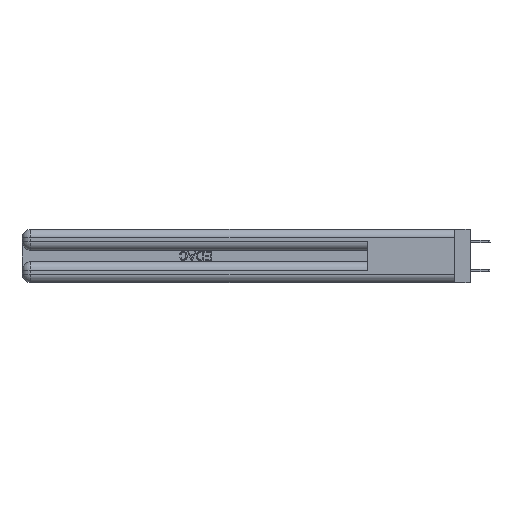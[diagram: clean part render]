
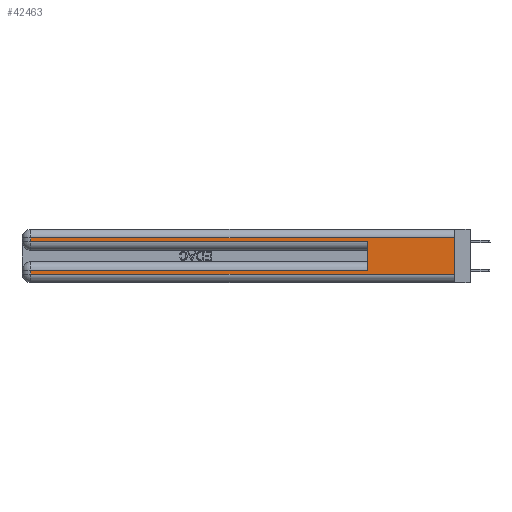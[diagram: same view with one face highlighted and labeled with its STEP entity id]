
A CAD part, left-side view. The second image highlights one B-rep face of the part: STEP entity #42463.
In plain terms, the highlighted planar face has unit normal (-1, 0, 0).
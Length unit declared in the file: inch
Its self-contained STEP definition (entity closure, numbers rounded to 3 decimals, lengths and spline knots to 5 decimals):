
#1510 = LINE ( 'NONE', #5532, #14162 ) ;
#2069 = VERTEX_POINT ( 'NONE', #32389 ) ;
#2329 = EDGE_CURVE ( 'NONE', #29139, #21231, #1510, .T. ) ;
#2401 = LINE ( 'NONE', #26599, #18452 ) ;
#2879 = PLANE ( 'NONE',  #22281 ) ;
#3464 = ORIENTED_EDGE ( 'NONE', *, *, #11914, .T. ) ;
#3567 = EDGE_CURVE ( 'NONE', #6010, #40529, #17371, .T. ) ;
#3738 = VECTOR ( 'NONE', #27726, 39.37008 ) ;
#5532 = CARTESIAN_POINT ( 'NONE',  ( 0., 0.6, 0.145 ) ) ;
#6010 = VERTEX_POINT ( 'NONE', #36579 ) ;
#7135 = ORIENTED_EDGE ( 'NONE', *, *, #15973, .T. ) ;
#7564 = LINE ( 'NONE', #41798, #3738 ) ;
#7764 = EDGE_LOOP ( 'NONE', ( #33104, #27864, #3464, #7135, #25531, #18415, #34031, #39210 ) ) ;
#7847 = LINE ( 'NONE', #17482, #26709 ) ;
#8867 = CARTESIAN_POINT ( 'NONE',  ( 0., 0., 0.06 ) ) ;
#9015 = DIRECTION ( 'NONE',  ( 0., 0., -1. ) ) ;
#10033 = EDGE_CURVE ( 'NONE', #29139, #22877, #33178, .T. ) ;
#10968 = DIRECTION ( 'NONE',  ( 0., -1., 0. ) ) ;
#11823 = DIRECTION ( 'NONE',  ( 0., 0., 1. ) ) ;
#11914 = EDGE_CURVE ( 'NONE', #40529, #38296, #33611, .T. ) ;
#12360 = LINE ( 'NONE', #15292, #13556 ) ;
#13556 = VECTOR ( 'NONE', #15062, 39.37008 ) ;
#13702 = CARTESIAN_POINT ( 'NONE',  ( 0., 2.94, 0.085 ) ) ;
#14162 = VECTOR ( 'NONE', #11823, 39.37008 ) ;
#14410 = VECTOR ( 'NONE', #9015, 39.37008 ) ;
#15062 = DIRECTION ( 'NONE',  ( 0., 0., -1. ) ) ;
#15292 = CARTESIAN_POINT ( 'NONE',  ( 0., 2.94, 0.37 ) ) ;
#15973 = EDGE_CURVE ( 'NONE', #38296, #21231, #7847, .T. ) ;
#16550 = DIRECTION ( 'NONE',  ( 0., 0., -1. ) ) ;
#17371 = LINE ( 'NONE', #34593, #29222 ) ;
#17482 = CARTESIAN_POINT ( 'NONE',  ( 0., 0., 0.285 ) ) ;
#18044 = DIRECTION ( 'NONE',  ( 0., 1., 0. ) ) ;
#18415 = ORIENTED_EDGE ( 'NONE', *, *, #10033, .T. ) ;
#18452 = VECTOR ( 'NONE', #19867, 39.37008 ) ;
#19053 = DIRECTION ( 'NONE',  ( 1., 0., 0. ) ) ;
#19692 = CARTESIAN_POINT ( 'NONE',  ( 0., 2.94, 0.31 ) ) ;
#19867 = DIRECTION ( 'NONE',  ( 0., -1., 0. ) ) ;
#21231 = VERTEX_POINT ( 'NONE', #33880 ) ;
#21248 = CARTESIAN_POINT ( 'NONE',  ( 0., 2.94, 0.285 ) ) ;
#22281 = AXIS2_PLACEMENT_3D ( 'NONE', #43193, #19053, #16550 ) ;
#22713 = CARTESIAN_POINT ( 'NONE',  ( 0., 0.6, 0.085 ) ) ;
#22877 = VERTEX_POINT ( 'NONE', #13702 ) ;
#24731 = CARTESIAN_POINT ( 'NONE',  ( 0., 0., 0.085 ) ) ;
#25531 = ORIENTED_EDGE ( 'NONE', *, *, #2329, .F. ) ;
#25563 = EDGE_CURVE ( 'NONE', #22877, #2069, #12360, .T. ) ;
#26050 = CARTESIAN_POINT ( 'NONE',  ( 0., 2.94, 0.37 ) ) ;
#26599 = CARTESIAN_POINT ( 'NONE',  ( 0., 0., 0.06 ) ) ;
#26709 = VECTOR ( 'NONE', #10968, 39.37008 ) ;
#27726 = DIRECTION ( 'NONE',  ( 0., 0., -1. ) ) ;
#27864 = ORIENTED_EDGE ( 'NONE', *, *, #3567, .T. ) ;
#29139 = VERTEX_POINT ( 'NONE', #22713 ) ;
#29222 = VECTOR ( 'NONE', #18044, 39.37008 ) ;
#32197 = VECTOR ( 'NONE', #38375, 39.37008 ) ;
#32389 = CARTESIAN_POINT ( 'NONE',  ( 0., 2.94, 0.06 ) ) ;
#33104 = ORIENTED_EDGE ( 'NONE', *, *, #43594, .F. ) ;
#33178 = LINE ( 'NONE', #24731, #32197 ) ;
#33555 = FACE_OUTER_BOUND ( 'NONE', #7764, .T. ) ;
#33611 = LINE ( 'NONE', #26050, #14410 ) ;
#33880 = CARTESIAN_POINT ( 'NONE',  ( 0., 0.6, 0.285 ) ) ;
#34031 = ORIENTED_EDGE ( 'NONE', *, *, #25563, .T. ) ;
#34593 = CARTESIAN_POINT ( 'NONE',  ( 0., 0., 0.31 ) ) ;
#35405 = EDGE_CURVE ( 'NONE', #2069, #37056, #2401, .T. ) ;
#36579 = CARTESIAN_POINT ( 'NONE',  ( 0., 0., 0.31 ) ) ;
#37056 = VERTEX_POINT ( 'NONE', #8867 ) ;
#38296 = VERTEX_POINT ( 'NONE', #21248 ) ;
#38375 = DIRECTION ( 'NONE',  ( 0., 1., 0. ) ) ;
#39210 = ORIENTED_EDGE ( 'NONE', *, *, #35405, .T. ) ;
#40529 = VERTEX_POINT ( 'NONE', #19692 ) ;
#41798 = CARTESIAN_POINT ( 'NONE',  ( 0., 0., 0.37 ) ) ;
#42463 = ADVANCED_FACE ( 'NONE', ( #33555 ), #2879, .F. ) ;
#43193 = CARTESIAN_POINT ( 'NONE',  ( 0., 0., 0.37 ) ) ;
#43594 = EDGE_CURVE ( 'NONE', #6010, #37056, #7564, .T. ) ;
